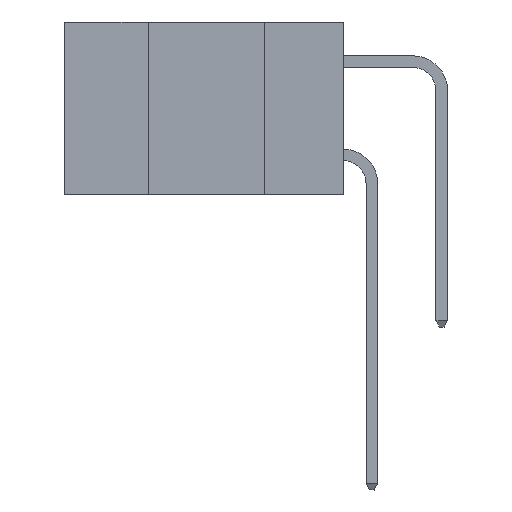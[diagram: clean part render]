
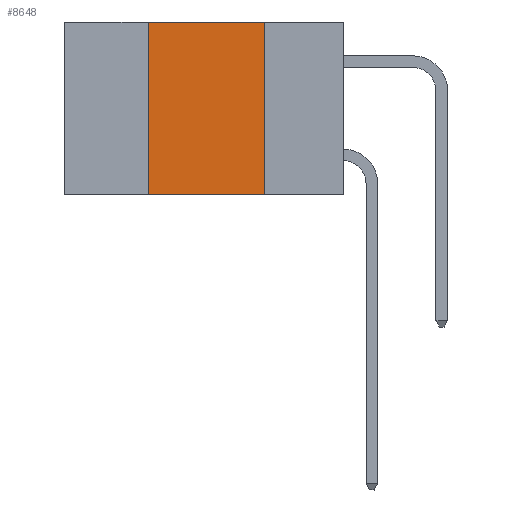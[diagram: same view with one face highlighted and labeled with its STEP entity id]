
A CAD part, left-side view. The second image highlights one B-rep face of the part: STEP entity #8648.
In plain terms, the highlighted planar face has unit normal (-1, 0, 0).
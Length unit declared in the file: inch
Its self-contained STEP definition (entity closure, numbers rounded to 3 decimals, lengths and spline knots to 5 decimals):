
#532 = DIRECTION ( 'NONE',  ( 0., -1., 0. ) ) ;
#1368 = CARTESIAN_POINT ( 'NONE',  ( 0., 0.42, 0. ) ) ;
#2049 = DIRECTION ( 'NONE',  ( 0., 0., 1. ) ) ;
#2083 = VECTOR ( 'NONE', #4934, 39.37008 ) ;
#4138 = VERTEX_POINT ( 'NONE', #19544 ) ;
#4366 = CARTESIAN_POINT ( 'NONE',  ( 0., 0.42, -0.37 ) ) ;
#4724 = CARTESIAN_POINT ( 'NONE',  ( 0., 0.17, -0.37 ) ) ;
#4934 = DIRECTION ( 'NONE',  ( 0., 0., -1. ) ) ;
#5267 = EDGE_LOOP ( 'NONE', ( #6482, #16826, #7309, #13424 ) ) ;
#5987 = DIRECTION ( 'NONE',  ( 0., 0., -1. ) ) ;
#5991 = DIRECTION ( 'NONE',  ( 0., -1., 0. ) ) ;
#6234 = CARTESIAN_POINT ( 'NONE',  ( 0., 0.6, 0. ) ) ;
#6346 = VERTEX_POINT ( 'NONE', #4724 ) ;
#6482 = ORIENTED_EDGE ( 'NONE', *, *, #13218, .F. ) ;
#7245 = EDGE_CURVE ( 'NONE', #7844, #6346, #17413, .T. ) ;
#7309 = ORIENTED_EDGE ( 'NONE', *, *, #17879, .F. ) ;
#7722 = VECTOR ( 'NONE', #2049, 39.37008 ) ;
#7844 = VERTEX_POINT ( 'NONE', #4366 ) ;
#8198 = CARTESIAN_POINT ( 'NONE',  ( 0., 0.6, -0.37 ) ) ;
#8648 = ADVANCED_FACE ( 'NONE', ( #9644 ), #19336, .F. ) ;
#8833 = CARTESIAN_POINT ( 'NONE',  ( 0., 0.17, -0.37 ) ) ;
#9272 = LINE ( 'NONE', #8833, #2083 ) ;
#9644 = FACE_OUTER_BOUND ( 'NONE', #5267, .T. ) ;
#9769 = CARTESIAN_POINT ( 'NONE',  ( 0., 0.6, 0. ) ) ;
#11772 = CARTESIAN_POINT ( 'NONE',  ( 0., 0.42, -0.37 ) ) ;
#13218 = EDGE_CURVE ( 'NONE', #4138, #6346, #9272, .T. ) ;
#13424 = ORIENTED_EDGE ( 'NONE', *, *, #7245, .T. ) ;
#14424 = AXIS2_PLACEMENT_3D ( 'NONE', #9769, #17519, #5987 ) ;
#14436 = VECTOR ( 'NONE', #5991, 39.37008 ) ;
#15563 = EDGE_CURVE ( 'NONE', #21624, #4138, #17280, .T. ) ;
#16826 = ORIENTED_EDGE ( 'NONE', *, *, #15563, .F. ) ;
#17037 = VECTOR ( 'NONE', #532, 39.37008 ) ;
#17280 = LINE ( 'NONE', #6234, #14436 ) ;
#17413 = LINE ( 'NONE', #8198, #17037 ) ;
#17519 = DIRECTION ( 'NONE',  ( 1., 0., 0. ) ) ;
#17879 = EDGE_CURVE ( 'NONE', #7844, #21624, #18685, .T. ) ;
#18685 = LINE ( 'NONE', #11772, #7722 ) ;
#19336 = PLANE ( 'NONE',  #14424 ) ;
#19544 = CARTESIAN_POINT ( 'NONE',  ( 0., 0.17, 0. ) ) ;
#21624 = VERTEX_POINT ( 'NONE', #1368 ) ;
